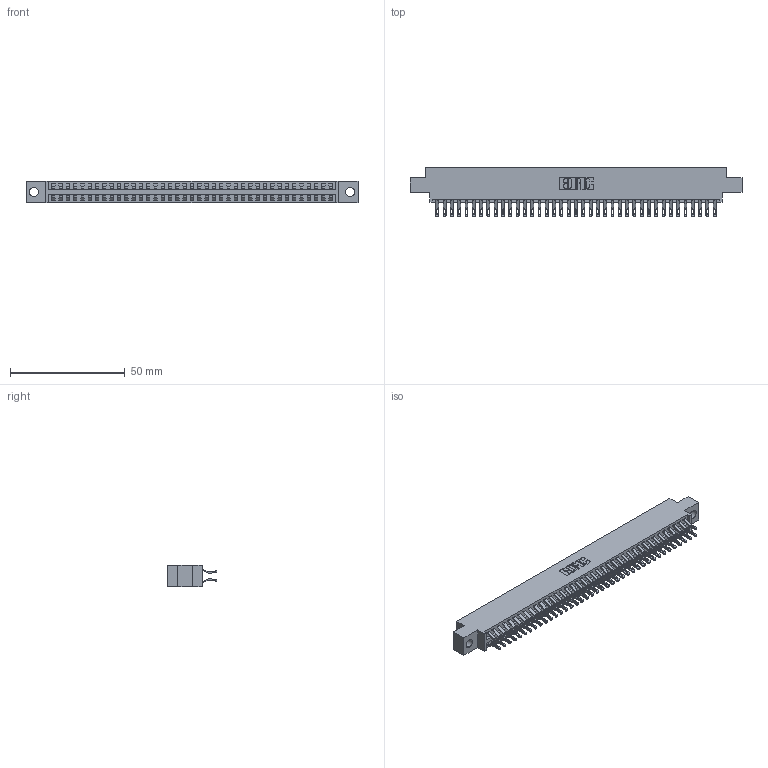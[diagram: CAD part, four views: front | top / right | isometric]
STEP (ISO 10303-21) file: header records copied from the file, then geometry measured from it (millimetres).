
FILE_DESCRIPTION (( 'STEP AP203' ), '1' );
FILE_NAME ('346-078-555-804.STEP', '2022-05-25T14:25:01', ( '' ), ( '' ), 'SwSTEP 2.0', 'SolidWorks 2020', '' );
FILE_SCHEMA (( 'CONFIG_CONTROL_DESIGN' ));
Length unit declared in the file: inch
Products named in the file (3): 345-292-001_555 Tail; 346-078-555-804; 346 Part_0.170 Offset - 0.156 Dia-TH
Assembly tree (79 placements, depth 2):
  346-078-555-804
    346 Part_0.170 Offset - 0.156 Dia-TH
    345-292-001_555 Tail  x78
Bounding box: 144.4 x 21.46 x 9.4 mm (x, y, z)
Volume: 14023.1 mm3; surface area: 20062.5 mm2
Topology: 79 solids, 79 shells, 4664 faces, 14651 edges, 9766 vertices
Faces by surface type: plane 2668, cylinder 1996
Entity records: 26733 total; most frequent: CARTESIAN_POINT 4452, ORIENTED_EDGE 4354, DIRECTION 3941, EDGE_CURVE 2177, LINE 1869, VECTOR 1869, VERTEX_POINT 1450, AXIS2_PLACEMENT_3D 1036
